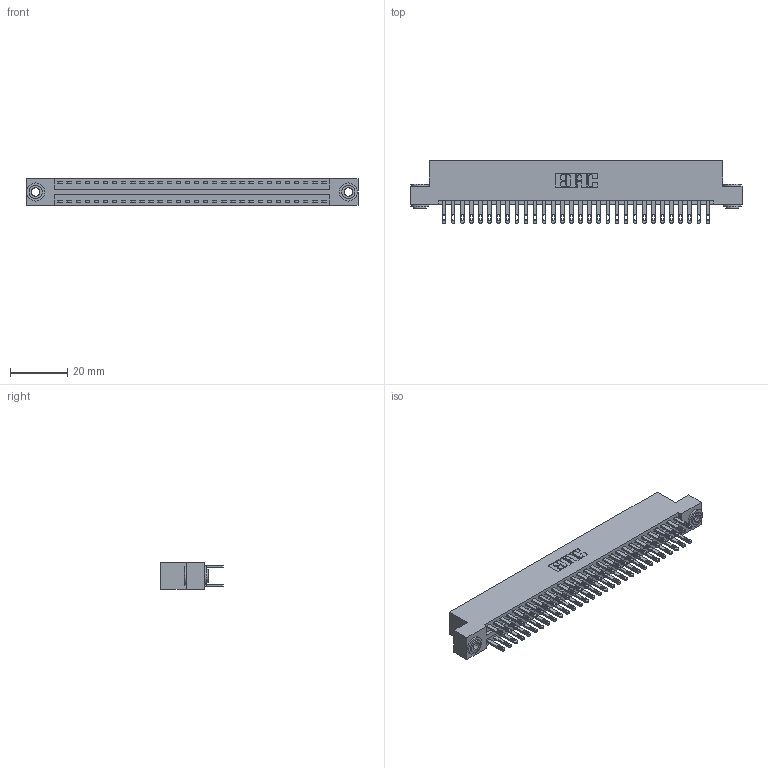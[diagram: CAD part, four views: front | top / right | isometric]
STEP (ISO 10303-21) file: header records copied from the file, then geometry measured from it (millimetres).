
FILE_DESCRIPTION (( 'STEP AP203' ), '1' );
FILE_NAME ('346-060-500-203.STEP', '2022-05-21T10:03:42', ( '' ), ( '' ), 'SwSTEP 2.0', 'SolidWorks 2020', '' );
FILE_SCHEMA (( 'CONFIG_CONTROL_DESIGN' ));
Length unit declared in the file: inch
Products named in the file (4): 345-250-002_345-250-002-102; 345-292-001_345-293-100; 346-060-500-203; 346 Part_Flush Mounting Lugs - 0.156 Dia-TH
Assembly tree (63 placements, depth 2):
  346-060-500-203
    346 Part_Flush Mounting Lugs - 0.156 Dia-TH
    345-292-001_345-293-100  x60
    345-250-002_345-250-002-102  x2
Bounding box: 115.82 x 21.84 x 9.4 mm (x, y, z)
Volume: 11385.7 mm3; surface area: 16338.5 mm2
Topology: 63 solids, 63 shells, 3054 faces, 9261 edges, 6170 vertices
Faces by surface type: plane 1840, cylinder 1206, cone 8
Entity records: 22190 total; most frequent: CARTESIAN_POINT 3653, ORIENTED_EDGE 3578, DIRECTION 3303, EDGE_CURVE 1789, LINE 1509, VECTOR 1509, VERTEX_POINT 1190, AXIS2_PLACEMENT_3D 897
